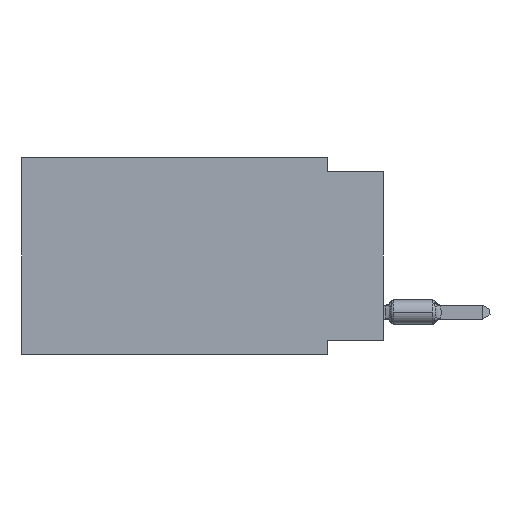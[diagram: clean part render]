
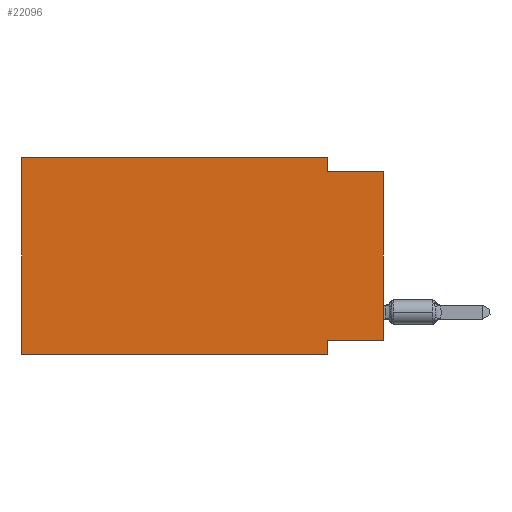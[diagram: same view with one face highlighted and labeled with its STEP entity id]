
A CAD part, left-side view. The second image highlights one B-rep face of the part: STEP entity #22096.
In plain terms, the highlighted planar face has unit normal (-1, 0, 0).
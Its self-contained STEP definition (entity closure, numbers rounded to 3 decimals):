
#473 = PLANE ( 'NONE',  #8991 ) ;
#549 = EDGE_CURVE ( 'NONE', #3972, #7689, #21856, .T. ) ;
#1158 = EDGE_LOOP ( 'NONE', ( #13648, #21008, #13924, #22635, #20734, #27401, #23105, #29504 ) ) ;
#1732 = VERTEX_POINT ( 'NONE', #30344 ) ;
#2092 = EDGE_CURVE ( 'NONE', #11959, #3972, #18229, .T. ) ;
#2568 = EDGE_CURVE ( 'NONE', #1732, #12049, #14273, .T. ) ;
#3151 = DIRECTION ( 'NONE',  ( 0., 0., 1. ) ) ;
#3972 = VERTEX_POINT ( 'NONE', #13129 ) ;
#4090 = DIRECTION ( 'NONE',  ( 0., 0., -1. ) ) ;
#4389 = CARTESIAN_POINT ( 'NONE',  ( 0., 2.54, -8.89 ) ) ;
#4549 = DIRECTION ( 'NONE',  ( 0., -1., 0. ) ) ;
#5028 = VERTEX_POINT ( 'NONE', #27756 ) ;
#6031 = CARTESIAN_POINT ( 'NONE',  ( 0., 16.383, -8.89 ) ) ;
#6928 = LINE ( 'NONE', #21912, #14142 ) ;
#7558 = CARTESIAN_POINT ( 'NONE',  ( 0., 2.54, -0.635 ) ) ;
#7679 = CARTESIAN_POINT ( 'NONE',  ( 0., 16.383, -8.89 ) ) ;
#7689 = VERTEX_POINT ( 'NONE', #7558 ) ;
#8506 = EDGE_CURVE ( 'NONE', #7689, #20926, #6928, .T. ) ;
#8582 = DIRECTION ( 'NONE',  ( 0., 0., 1. ) ) ;
#8672 = VECTOR ( 'NONE', #29799, 1000. ) ;
#8991 = AXIS2_PLACEMENT_3D ( 'NONE', #29756, #15454, #19904 ) ;
#10333 = FACE_OUTER_BOUND ( 'NONE', #1158, .T. ) ;
#10743 = CARTESIAN_POINT ( 'NONE',  ( 0., 16.383, 0. ) ) ;
#11748 = VECTOR ( 'NONE', #4090, 1000. ) ;
#11959 = VERTEX_POINT ( 'NONE', #13252 ) ;
#12049 = VERTEX_POINT ( 'NONE', #14189 ) ;
#12296 = EDGE_CURVE ( 'NONE', #23285, #11959, #27358, .T. ) ;
#13129 = CARTESIAN_POINT ( 'NONE',  ( 0., 2.54, 0. ) ) ;
#13252 = CARTESIAN_POINT ( 'NONE',  ( 0., 16.383, 0. ) ) ;
#13648 = ORIENTED_EDGE ( 'NONE', *, *, #23384, .T. ) ;
#13924 = ORIENTED_EDGE ( 'NONE', *, *, #549, .F. ) ;
#14142 = VECTOR ( 'NONE', #4549, 1000. ) ;
#14189 = CARTESIAN_POINT ( 'NONE',  ( 0., 2.54, -8.255 ) ) ;
#14273 = LINE ( 'NONE', #16970, #17781 ) ;
#14538 = DIRECTION ( 'NONE',  ( 0., 0., -1. ) ) ;
#15289 = CARTESIAN_POINT ( 'NONE',  ( 0., 16.383, 0. ) ) ;
#15454 = DIRECTION ( 'NONE',  ( 1., 0., 0. ) ) ;
#16498 = DIRECTION ( 'NONE',  ( 0., 1., 0. ) ) ;
#16718 = EDGE_CURVE ( 'NONE', #12049, #5028, #18755, .T. ) ;
#16970 = CARTESIAN_POINT ( 'NONE',  ( 0., 0., -8.255 ) ) ;
#17738 = EDGE_CURVE ( 'NONE', #23285, #5028, #20089, .T. ) ;
#17781 = VECTOR ( 'NONE', #16498, 1000. ) ;
#18229 = LINE ( 'NONE', #10743, #22835 ) ;
#18755 = LINE ( 'NONE', #4389, #11748 ) ;
#18979 = VECTOR ( 'NONE', #14538, 1000. ) ;
#19904 = DIRECTION ( 'NONE',  ( 0., 0., -1. ) ) ;
#20089 = LINE ( 'NONE', #7679, #8672 ) ;
#20734 = ORIENTED_EDGE ( 'NONE', *, *, #12296, .F. ) ;
#20791 = CARTESIAN_POINT ( 'NONE',  ( 0., 2.54, 0. ) ) ;
#20926 = VERTEX_POINT ( 'NONE', #29972 ) ;
#21008 = ORIENTED_EDGE ( 'NONE', *, *, #8506, .F. ) ;
#21856 = LINE ( 'NONE', #20791, #18979 ) ;
#21912 = CARTESIAN_POINT ( 'NONE',  ( 0., 0., -0.635 ) ) ;
#22096 = ADVANCED_FACE ( 'NONE', ( #10333 ), #473, .F. ) ;
#22273 = VECTOR ( 'NONE', #8582, 1000. ) ;
#22635 = ORIENTED_EDGE ( 'NONE', *, *, #2092, .F. ) ;
#22835 = VECTOR ( 'NONE', #27613, 1000. ) ;
#23105 = ORIENTED_EDGE ( 'NONE', *, *, #16718, .F. ) ;
#23285 = VERTEX_POINT ( 'NONE', #6031 ) ;
#23384 = EDGE_CURVE ( 'NONE', #1732, #20926, #25764, .T. ) ;
#25475 = CARTESIAN_POINT ( 'NONE',  ( 0., 0., 0. ) ) ;
#25764 = LINE ( 'NONE', #25475, #22273 ) ;
#27358 = LINE ( 'NONE', #15289, #30427 ) ;
#27401 = ORIENTED_EDGE ( 'NONE', *, *, #17738, .T. ) ;
#27613 = DIRECTION ( 'NONE',  ( 0., -1., 0. ) ) ;
#27756 = CARTESIAN_POINT ( 'NONE',  ( 0., 2.54, -8.89 ) ) ;
#29504 = ORIENTED_EDGE ( 'NONE', *, *, #2568, .F. ) ;
#29756 = CARTESIAN_POINT ( 'NONE',  ( 0., 16.383, 0. ) ) ;
#29799 = DIRECTION ( 'NONE',  ( 0., -1., 0. ) ) ;
#29972 = CARTESIAN_POINT ( 'NONE',  ( 0., 0., -0.635 ) ) ;
#30344 = CARTESIAN_POINT ( 'NONE',  ( 0., 0., -8.255 ) ) ;
#30427 = VECTOR ( 'NONE', #3151, 1000. ) ;
